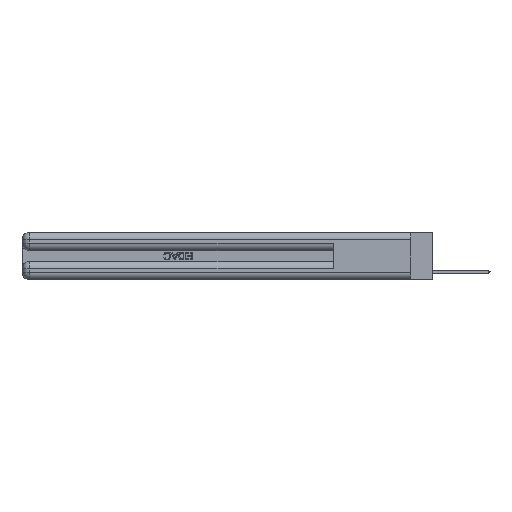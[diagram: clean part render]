
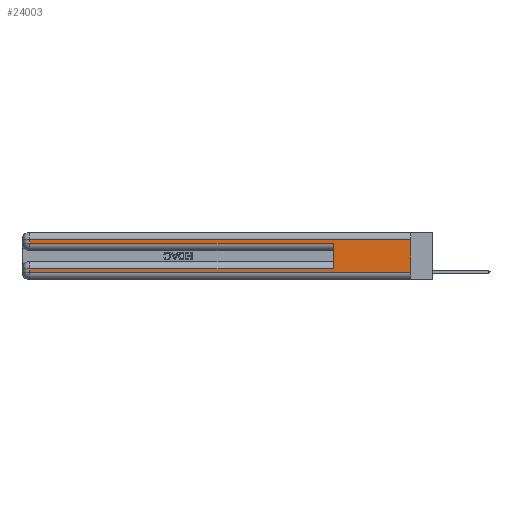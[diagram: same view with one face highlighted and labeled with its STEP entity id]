
A CAD part, left-side view. The second image highlights one B-rep face of the part: STEP entity #24003.
In plain terms, the highlighted planar face has unit normal (-1, 0, 0).
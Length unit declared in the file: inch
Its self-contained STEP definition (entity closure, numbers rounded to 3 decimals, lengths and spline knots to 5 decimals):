
#1062 = VERTEX_POINT ( 'NONE', #6534 ) ;
#1495 = CARTESIAN_POINT ( 'NONE',  ( 0., 0., 0.31 ) ) ;
#1866 = DIRECTION ( 'NONE',  ( 0., 1., 0. ) ) ;
#2112 = ORIENTED_EDGE ( 'NONE', *, *, #10536, .T. ) ;
#3385 = VERTEX_POINT ( 'NONE', #11223 ) ;
#3609 = DIRECTION ( 'NONE',  ( 0., -1., 0. ) ) ;
#3849 = VECTOR ( 'NONE', #16132, 39.37008 ) ;
#4362 = EDGE_CURVE ( 'NONE', #7836, #18046, #19536, .T. ) ;
#5560 = LINE ( 'NONE', #24284, #3849 ) ;
#6219 = VERTEX_POINT ( 'NONE', #11586 ) ;
#6369 = ORIENTED_EDGE ( 'NONE', *, *, #13600, .T. ) ;
#6515 = FACE_OUTER_BOUND ( 'NONE', #22184, .T. ) ;
#6534 = CARTESIAN_POINT ( 'NONE',  ( 0., 0.6, 0.285 ) ) ;
#7438 = CARTESIAN_POINT ( 'NONE',  ( 0., 0., 0.085 ) ) ;
#7547 = DIRECTION ( 'NONE',  ( 0., 0., -1. ) ) ;
#7741 = DIRECTION ( 'NONE',  ( 0., 0., -1. ) ) ;
#7836 = VERTEX_POINT ( 'NONE', #30252 ) ;
#8435 = CARTESIAN_POINT ( 'NONE',  ( 0., 0., 0.06 ) ) ;
#8609 = LINE ( 'NONE', #19925, #13263 ) ;
#9342 = LINE ( 'NONE', #27703, #33984 ) ;
#10536 = EDGE_CURVE ( 'NONE', #14432, #35211, #14418, .T. ) ;
#11223 = CARTESIAN_POINT ( 'NONE',  ( 0., 2.94, 0.285 ) ) ;
#11452 = VECTOR ( 'NONE', #19389, 39.37008 ) ;
#11586 = CARTESIAN_POINT ( 'NONE',  ( 0., 2.94, 0.31 ) ) ;
#12003 = LINE ( 'NONE', #7438, #29907 ) ;
#12212 = DIRECTION ( 'NONE',  ( 0., 1., 0. ) ) ;
#12339 = DIRECTION ( 'NONE',  ( 0., 0., -1. ) ) ;
#12866 = VECTOR ( 'NONE', #12212, 39.37008 ) ;
#13263 = VECTOR ( 'NONE', #3609, 39.37008 ) ;
#13352 = ORIENTED_EDGE ( 'NONE', *, *, #13576, .T. ) ;
#13576 = EDGE_CURVE ( 'NONE', #7836, #6219, #26483, .T. ) ;
#13600 = EDGE_CURVE ( 'NONE', #26120, #14432, #12003, .T. ) ;
#14418 = LINE ( 'NONE', #23839, #25965 ) ;
#14432 = VERTEX_POINT ( 'NONE', #22744 ) ;
#15388 = CARTESIAN_POINT ( 'NONE',  ( 0., 0., 0.37 ) ) ;
#16132 = DIRECTION ( 'NONE',  ( 0., 0., 1. ) ) ;
#17560 = CARTESIAN_POINT ( 'NONE',  ( 0., 2.94, 0.37 ) ) ;
#18046 = VERTEX_POINT ( 'NONE', #8435 ) ;
#18506 = DIRECTION ( 'NONE',  ( 1., 0., 0. ) ) ;
#18658 = EDGE_CURVE ( 'NONE', #35211, #18046, #8609, .T. ) ;
#19389 = DIRECTION ( 'NONE',  ( 0., 0., -1. ) ) ;
#19536 = LINE ( 'NONE', #32923, #11452 ) ;
#19925 = CARTESIAN_POINT ( 'NONE',  ( 0., 0., 0.06 ) ) ;
#20211 = EDGE_CURVE ( 'NONE', #26120, #1062, #5560, .T. ) ;
#21101 = EDGE_CURVE ( 'NONE', #3385, #1062, #9342, .T. ) ;
#22184 = EDGE_LOOP ( 'NONE', ( #29405, #13352, #34821, #28139, #24045, #6369, #2112, #24881 ) ) ;
#22744 = CARTESIAN_POINT ( 'NONE',  ( 0., 2.94, 0.085 ) ) ;
#23651 = EDGE_CURVE ( 'NONE', #6219, #3385, #25363, .T. ) ;
#23839 = CARTESIAN_POINT ( 'NONE',  ( 0., 2.94, 0.37 ) ) ;
#23873 = PLANE ( 'NONE',  #33126 ) ;
#24003 = ADVANCED_FACE ( 'NONE', ( #6515 ), #23873, .F. ) ;
#24045 = ORIENTED_EDGE ( 'NONE', *, *, #20211, .F. ) ;
#24284 = CARTESIAN_POINT ( 'NONE',  ( 0., 0.6, 0.145 ) ) ;
#24500 = VECTOR ( 'NONE', #12339, 39.37008 ) ;
#24879 = DIRECTION ( 'NONE',  ( 0., -1., 0. ) ) ;
#24881 = ORIENTED_EDGE ( 'NONE', *, *, #18658, .T. ) ;
#25363 = LINE ( 'NONE', #17560, #24500 ) ;
#25674 = CARTESIAN_POINT ( 'NONE',  ( 0., 2.94, 0.06 ) ) ;
#25965 = VECTOR ( 'NONE', #7741, 39.37008 ) ;
#26120 = VERTEX_POINT ( 'NONE', #29939 ) ;
#26483 = LINE ( 'NONE', #1495, #12866 ) ;
#27703 = CARTESIAN_POINT ( 'NONE',  ( 0., 0., 0.285 ) ) ;
#28139 = ORIENTED_EDGE ( 'NONE', *, *, #21101, .T. ) ;
#29405 = ORIENTED_EDGE ( 'NONE', *, *, #4362, .F. ) ;
#29907 = VECTOR ( 'NONE', #1866, 39.37008 ) ;
#29939 = CARTESIAN_POINT ( 'NONE',  ( 0., 0.6, 0.085 ) ) ;
#30252 = CARTESIAN_POINT ( 'NONE',  ( 0., 0., 0.31 ) ) ;
#32923 = CARTESIAN_POINT ( 'NONE',  ( 0., 0., 0.37 ) ) ;
#33126 = AXIS2_PLACEMENT_3D ( 'NONE', #15388, #18506, #7547 ) ;
#33984 = VECTOR ( 'NONE', #24879, 39.37008 ) ;
#34821 = ORIENTED_EDGE ( 'NONE', *, *, #23651, .T. ) ;
#35211 = VERTEX_POINT ( 'NONE', #25674 ) ;
